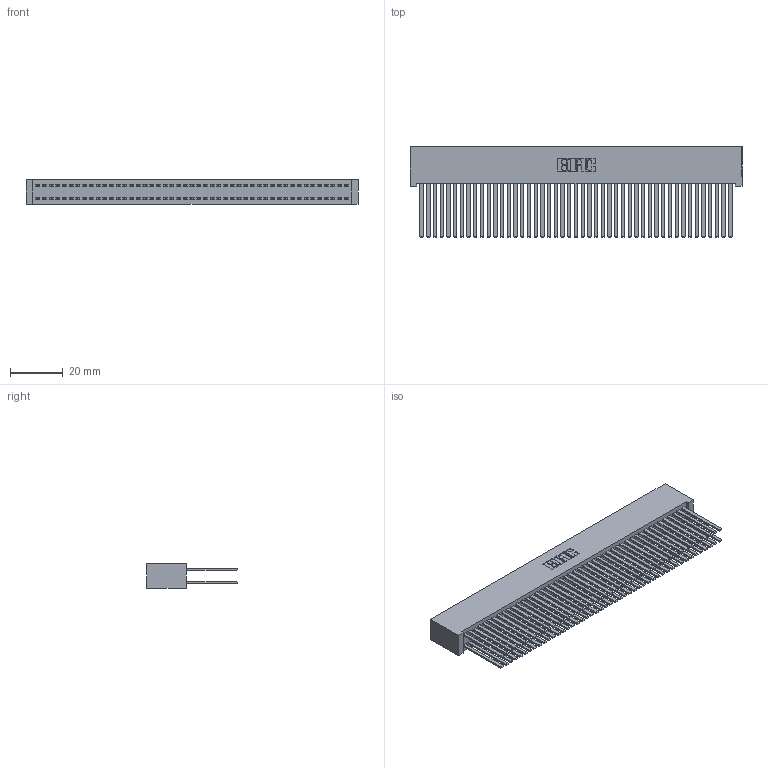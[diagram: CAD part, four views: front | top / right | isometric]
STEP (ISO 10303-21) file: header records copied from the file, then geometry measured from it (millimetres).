
FILE_DESCRIPTION (( 'STEP AP203' ), '1' );
FILE_NAME ('392-094-544-201.STEP', '2019-10-09T19:26:33', ( '' ), ( '' ), 'SwSTEP 2.0', 'SolidWorks 2016', '' );
FILE_SCHEMA (( 'CONFIG_CONTROL_DESIGN' ));
Length unit declared in the file: inch
Products named in the file (3): 342 Part_Lugless; 345-292-001_345-293-144; 392-094-544-201
Assembly tree (95 placements, depth 2):
  392-094-544-201
    342 Part_Lugless
    345-292-001_345-293-144  x94
Bounding box: 125.63 x 34.3 x 9.4 mm (x, y, z)
Volume: 13068.6 mm3; surface area: 25491 mm2
Topology: 95 solids, 95 shells, 4426 faces, 13153 edges, 8642 vertices
Faces by surface type: plane 3070, cylinder 1356
Entity records: 28997 total; most frequent: CARTESIAN_POINT 4794, ORIENTED_EDGE 4730, DIRECTION 4077, EDGE_CURVE 2365, VECTOR 2249, LINE 2249, VERTEX_POINT 1574, AXIS2_PLACEMENT_3D 914
